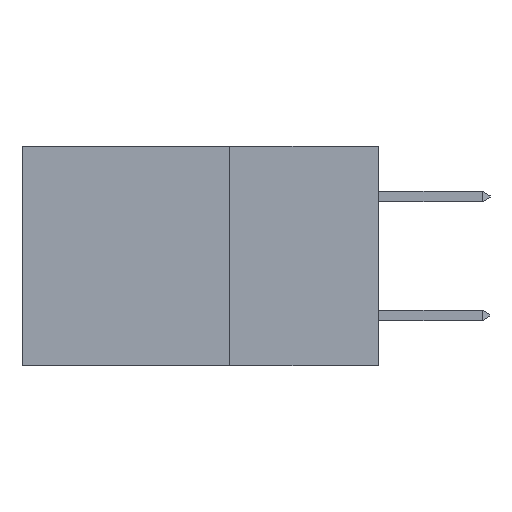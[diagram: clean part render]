
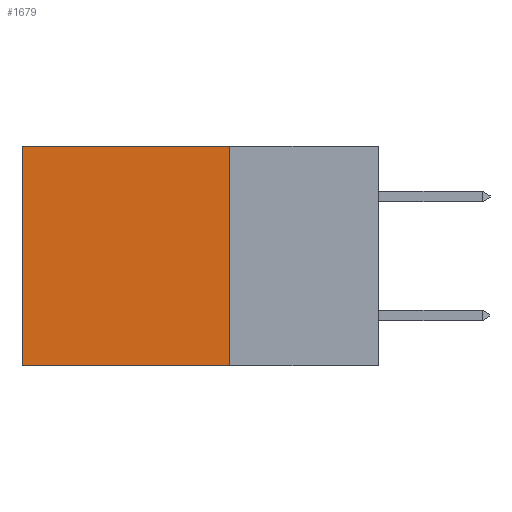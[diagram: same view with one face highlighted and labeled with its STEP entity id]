
A CAD part, left-side view. The second image highlights one B-rep face of the part: STEP entity #1679.
In plain terms, the highlighted planar face has unit normal (-1, 0, 0).
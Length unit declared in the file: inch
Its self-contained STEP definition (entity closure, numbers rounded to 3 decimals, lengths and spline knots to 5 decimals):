
#474 = DIRECTION ( 'NONE',  ( 0., 0., -1. ) ) ;
#579 = EDGE_CURVE ( 'NONE', #1049, #3846, #1442, .T. ) ;
#760 = VECTOR ( 'NONE', #3253, 39.37008 ) ;
#807 = CARTESIAN_POINT ( 'NONE',  ( 0.298, 0.25, 0. ) ) ;
#1049 = VERTEX_POINT ( 'NONE', #2814 ) ;
#1212 = LINE ( 'NONE', #807, #3865 ) ;
#1442 = LINE ( 'NONE', #6829, #8728 ) ;
#1670 = DIRECTION ( 'NONE',  ( 0., 0., -1. ) ) ;
#1679 = ADVANCED_FACE ( 'NONE', ( #10544 ), #5425, .F. ) ;
#1783 = ORIENTED_EDGE ( 'NONE', *, *, #5223, .F. ) ;
#1992 = CARTESIAN_POINT ( 'NONE',  ( 0.298, 0.25, 0. ) ) ;
#2814 = CARTESIAN_POINT ( 'NONE',  ( 0.298, 0.6, 0. ) ) ;
#3137 = LINE ( 'NONE', #1992, #760 ) ;
#3253 = DIRECTION ( 'NONE',  ( 0., 1., 0. ) ) ;
#3846 = VERTEX_POINT ( 'NONE', #10682 ) ;
#3865 = VECTOR ( 'NONE', #474, 39.37008 ) ;
#4441 = DIRECTION ( 'NONE',  ( 0., 0., -1. ) ) ;
#5223 = EDGE_CURVE ( 'NONE', #7612, #3846, #10592, .T. ) ;
#5425 = PLANE ( 'NONE',  #8973 ) ;
#5433 = EDGE_LOOP ( 'NONE', ( #11149, #1783, #6715, #8996 ) ) ;
#5495 = DIRECTION ( 'NONE',  ( 0., 1., 0. ) ) ;
#5549 = DIRECTION ( 'NONE',  ( 1., 0., 0. ) ) ;
#5584 = CARTESIAN_POINT ( 'NONE',  ( 0.298, 0.25, 0. ) ) ;
#5946 = CARTESIAN_POINT ( 'NONE',  ( 0.298, 0.25, -0.37 ) ) ;
#6292 = CARTESIAN_POINT ( 'NONE',  ( 0.298, 0.25, -0.37 ) ) ;
#6599 = EDGE_CURVE ( 'NONE', #9872, #1049, #3137, .T. ) ;
#6715 = ORIENTED_EDGE ( 'NONE', *, *, #9068, .F. ) ;
#6829 = CARTESIAN_POINT ( 'NONE',  ( 0.298, 0.6, 0. ) ) ;
#7612 = VERTEX_POINT ( 'NONE', #5946 ) ;
#8188 = VECTOR ( 'NONE', #5495, 39.37008 ) ;
#8728 = VECTOR ( 'NONE', #1670, 39.37008 ) ;
#8973 = AXIS2_PLACEMENT_3D ( 'NONE', #5584, #5549, #4441 ) ;
#8996 = ORIENTED_EDGE ( 'NONE', *, *, #6599, .T. ) ;
#9067 = CARTESIAN_POINT ( 'NONE',  ( 0.298, 0.25, 0. ) ) ;
#9068 = EDGE_CURVE ( 'NONE', #9872, #7612, #1212, .T. ) ;
#9872 = VERTEX_POINT ( 'NONE', #9067 ) ;
#10544 = FACE_OUTER_BOUND ( 'NONE', #5433, .T. ) ;
#10592 = LINE ( 'NONE', #6292, #8188 ) ;
#10682 = CARTESIAN_POINT ( 'NONE',  ( 0.298, 0.6, -0.37 ) ) ;
#11149 = ORIENTED_EDGE ( 'NONE', *, *, #579, .T. ) ;
